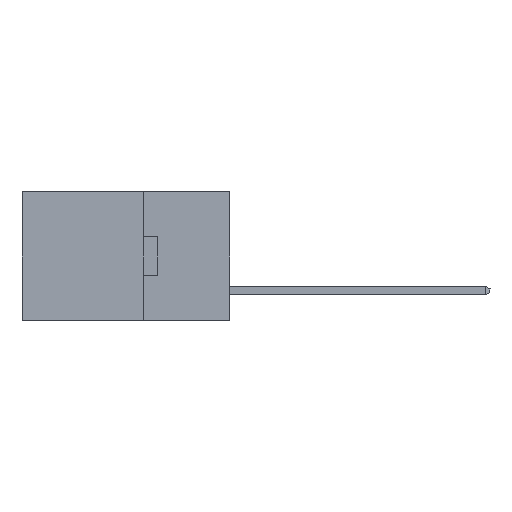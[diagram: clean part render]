
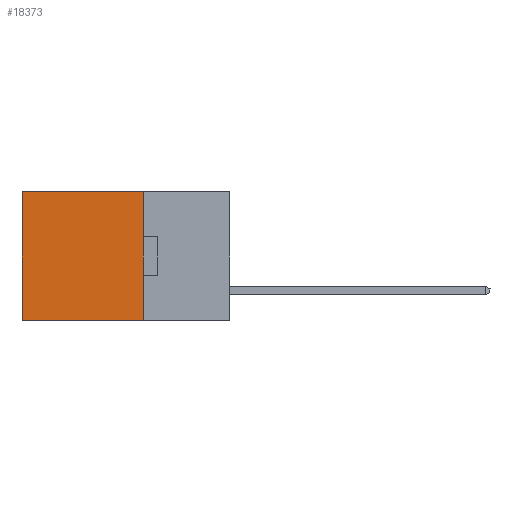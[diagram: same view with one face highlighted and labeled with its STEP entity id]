
A CAD part, left-side view. The second image highlights one B-rep face of the part: STEP entity #18373.
In plain terms, the highlighted planar face has unit normal (-1, 0, 0).
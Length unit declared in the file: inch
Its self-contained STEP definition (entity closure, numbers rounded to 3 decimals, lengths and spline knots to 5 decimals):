
#1266 = DIRECTION ( 'NONE',  ( 1., 0., 0. ) ) ;
#1601 = VECTOR ( 'NONE', #2772, 39.37008 ) ;
#2772 = DIRECTION ( 'NONE',  ( 0., 0., -1. ) ) ;
#3095 = ORIENTED_EDGE ( 'NONE', *, *, #13575, .F. ) ;
#3750 = EDGE_CURVE ( 'NONE', #18630, #12362, #15768, .T. ) ;
#3792 = ORIENTED_EDGE ( 'NONE', *, *, #3750, .T. ) ;
#3841 = DIRECTION ( 'NONE',  ( 0., 0., -1. ) ) ;
#4189 = CARTESIAN_POINT ( 'NONE',  ( 0.2615, 0.25, -0.37 ) ) ;
#4476 = ORIENTED_EDGE ( 'NONE', *, *, #14968, .T. ) ;
#4951 = CARTESIAN_POINT ( 'NONE',  ( 0.2615, 0.6, -0.37 ) ) ;
#5619 = CARTESIAN_POINT ( 'NONE',  ( 0.2615, 0.25, -0.37 ) ) ;
#6559 = EDGE_CURVE ( 'NONE', #18630, #24283, #23490, .T. ) ;
#6934 = AXIS2_PLACEMENT_3D ( 'NONE', #5619, #1266, #3841 ) ;
#7123 = CARTESIAN_POINT ( 'NONE',  ( 0.2615, 0.25, 0. ) ) ;
#7552 = CARTESIAN_POINT ( 'NONE',  ( 0.2615, 0.6, 0. ) ) ;
#7710 = VECTOR ( 'NONE', #17323, 39.37008 ) ;
#7798 = VERTEX_POINT ( 'NONE', #21623 ) ;
#8593 = LINE ( 'NONE', #25482, #7710 ) ;
#12362 = VERTEX_POINT ( 'NONE', #7552 ) ;
#13575 = EDGE_CURVE ( 'NONE', #24283, #7798, #8593, .T. ) ;
#14968 = EDGE_CURVE ( 'NONE', #12362, #7798, #15440, .T. ) ;
#15300 = CARTESIAN_POINT ( 'NONE',  ( 0.2615, 0.25, -0.37 ) ) ;
#15309 = VECTOR ( 'NONE', #22316, 39.37008 ) ;
#15440 = LINE ( 'NONE', #4951, #1601 ) ;
#15768 = LINE ( 'NONE', #16026, #15309 ) ;
#16026 = CARTESIAN_POINT ( 'NONE',  ( 0.2615, 0.25, 0. ) ) ;
#16818 = ORIENTED_EDGE ( 'NONE', *, *, #6559, .F. ) ;
#17323 = DIRECTION ( 'NONE',  ( 0., 1., 0. ) ) ;
#18373 = ADVANCED_FACE ( 'NONE', ( #24567 ), #24297, .F. ) ;
#18630 = VERTEX_POINT ( 'NONE', #7123 ) ;
#21328 = EDGE_LOOP ( 'NONE', ( #4476, #3095, #16818, #3792 ) ) ;
#21462 = DIRECTION ( 'NONE',  ( 0., 0., -1. ) ) ;
#21623 = CARTESIAN_POINT ( 'NONE',  ( 0.2615, 0.6, -0.37 ) ) ;
#22316 = DIRECTION ( 'NONE',  ( 0., 1., 0. ) ) ;
#23490 = LINE ( 'NONE', #15300, #23638 ) ;
#23638 = VECTOR ( 'NONE', #21462, 39.37008 ) ;
#24283 = VERTEX_POINT ( 'NONE', #4189 ) ;
#24297 = PLANE ( 'NONE',  #6934 ) ;
#24567 = FACE_OUTER_BOUND ( 'NONE', #21328, .T. ) ;
#25482 = CARTESIAN_POINT ( 'NONE',  ( 0.2615, 0.25, -0.37 ) ) ;
